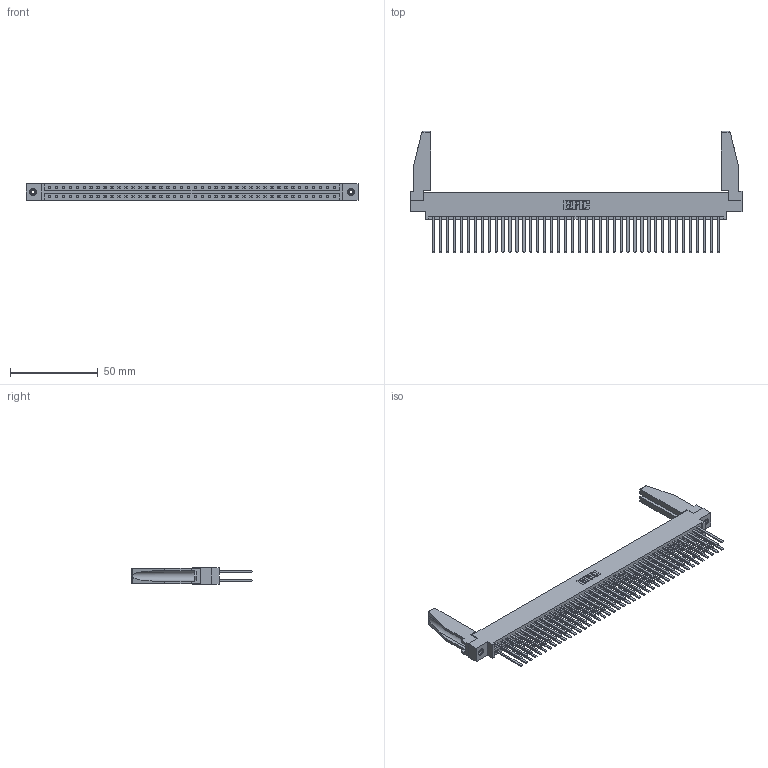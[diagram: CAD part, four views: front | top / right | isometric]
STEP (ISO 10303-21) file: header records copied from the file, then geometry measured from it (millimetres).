
FILE_DESCRIPTION (( 'STEP AP203' ), '1' );
FILE_NAME ('337-084-544-878.STEP', '2019-10-15T18:15:12', ( '' ), ( '' ), 'SwSTEP 2.0', 'SolidWorks 2016', '' );
FILE_SCHEMA (( 'CONFIG_CONTROL_DESIGN' ));
Length unit declared in the file: inch
Products named in the file (5): 345-250-001_345-250-001-102; 337 Part_0.170 Offset - 0.156 Dia-TI; 307-220-078; 345-292-001_345-293-144; 337-084-544-878
Assembly tree (89 placements, depth 2):
  337-084-544-878
    337 Part_0.170 Offset - 0.156 Dia-TI
    345-292-001_345-293-144  x84
    345-250-001_345-250-001-102  x2
    307-220-078  x2
Bounding box: 189.43 x 69.09 x 9.4 mm (x, y, z)
Volume: 25017.3 mm3; surface area: 31552.6 mm2
Topology: 89 solids, 89 shells, 4280 faces, 12665 edges, 8322 vertices
Faces by surface type: plane 3014, cylinder 1250, cone 12, torus 4
Entity records: 34952 total; most frequent: CARTESIAN_POINT 5888, ORIENTED_EDGE 5780, DIRECTION 5010, EDGE_CURVE 2890, VECTOR 2728, LINE 2728, VERTEX_POINT 1920, AXIS2_PLACEMENT_3D 1141
